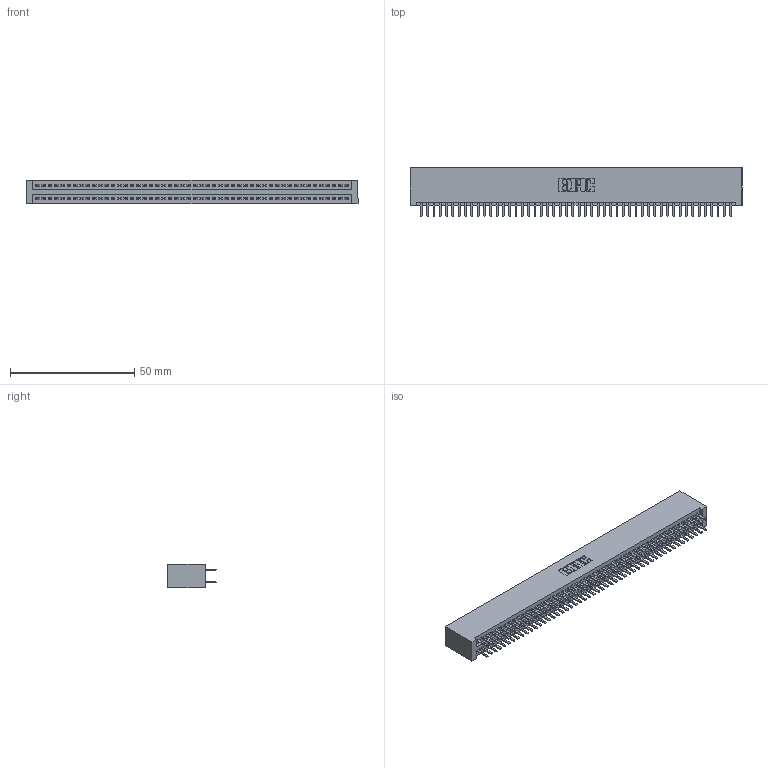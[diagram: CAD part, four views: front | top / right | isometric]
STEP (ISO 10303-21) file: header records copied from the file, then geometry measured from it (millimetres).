
FILE_DESCRIPTION (( 'STEP AP203' ), '1' );
FILE_NAME ('395-100-520-201.STEP', '2019-10-26T14:36:08', ( '' ), ( '' ), 'SwSTEP 2.0', 'SolidWorks 2016', '' );
FILE_SCHEMA (( 'CONFIG_CONTROL_DESIGN' ));
Length unit declared in the file: inch
Products named in the file (3): 345 Part_No Mounting Lugs; 345-292-001_345-293-120; 395-100-520-201
Assembly tree (101 placements, depth 2):
  395-100-520-201
    345 Part_No Mounting Lugs
    345-292-001_345-293-120  x100
Bounding box: 133.6 x 19.68 x 9.4 mm (x, y, z)
Volume: 13624.6 mm3; surface area: 20504.2 mm2
Topology: 101 solids, 101 shells, 5518 faces, 16017 edges, 10410 vertices
Faces by surface type: plane 3576, cylinder 1942
Entity records: 37991 total; most frequent: CARTESIAN_POINT 6372, ORIENTED_EDGE 6294, DIRECTION 5591, EDGE_CURVE 3147, VECTOR 2819, LINE 2819, VERTEX_POINT 2094, AXIS2_PLACEMENT_3D 1386
